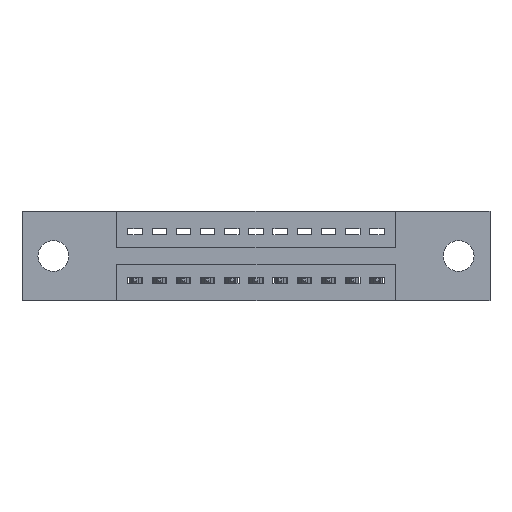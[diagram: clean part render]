
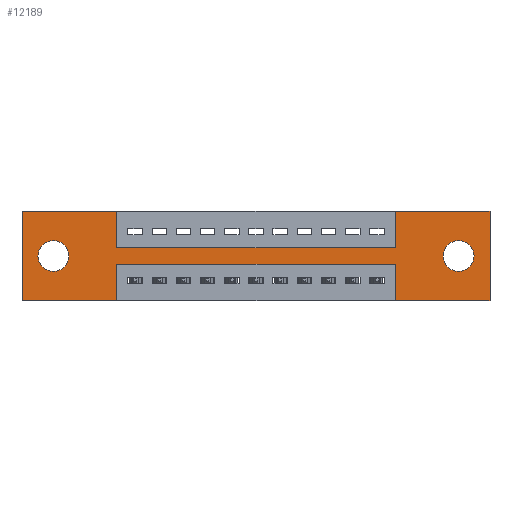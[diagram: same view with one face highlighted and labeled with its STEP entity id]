
A CAD part, front view. The second image highlights one B-rep face of the part: STEP entity #12189.
In plain terms, the highlighted planar face has unit normal (0, -1, 0).
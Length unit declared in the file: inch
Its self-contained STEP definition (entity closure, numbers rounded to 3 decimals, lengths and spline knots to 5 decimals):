
#134 = VERTEX_POINT ( 'NONE', #2562 ) ;
#169 = CARTESIAN_POINT ( 'NONE',  ( 0.3925, 0., -0.22 ) ) ;
#222 = DIRECTION ( 'NONE',  ( 0., 0., -1. ) ) ;
#341 = EDGE_CURVE ( 'NONE', #4711, #7004, #10070, .T. ) ;
#349 = ORIENTED_EDGE ( 'NONE', *, *, #8525, .F. ) ;
#428 = CARTESIAN_POINT ( 'NONE',  ( 1.935, 0., -0.37 ) ) ;
#443 = EDGE_LOOP ( 'NONE', ( #745, #349, #12490, #7075, #9271, #6505, #10443, #10310, #5885, #6499, #12311, #8963 ) ) ;
#560 = EDGE_CURVE ( 'NONE', #821, #6272, #3899, .T. ) ;
#649 = DIRECTION ( 'NONE',  ( 0., 0., 1. ) ) ;
#668 = CARTESIAN_POINT ( 'NONE',  ( 1.5425, 0., -0.37 ) ) ;
#745 = ORIENTED_EDGE ( 'NONE', *, *, #5936, .F. ) ;
#783 = DIRECTION ( 'NONE',  ( 0., 0., 1. ) ) ;
#821 = VERTEX_POINT ( 'NONE', #4050 ) ;
#855 = EDGE_CURVE ( 'NONE', #2214, #8982, #4069, .T. ) ;
#941 = AXIS2_PLACEMENT_3D ( 'NONE', #1010, #11714, #4969 ) ;
#1010 = CARTESIAN_POINT ( 'NONE',  ( 0.13, 0., -0.185 ) ) ;
#1178 = EDGE_CURVE ( 'NONE', #4798, #1387, #4210, .T. ) ;
#1194 = LINE ( 'NONE', #11105, #7691 ) ;
#1252 = VECTOR ( 'NONE', #10037, 39.37008 ) ;
#1342 = VECTOR ( 'NONE', #5977, 39.37008 ) ;
#1387 = VERTEX_POINT ( 'NONE', #1488 ) ;
#1488 = CARTESIAN_POINT ( 'NONE',  ( 1.5425, 0., 0. ) ) ;
#1522 = DIRECTION ( 'NONE',  ( 1., 0., 0. ) ) ;
#1753 = CARTESIAN_POINT ( 'NONE',  ( 1.5425, 0., 0. ) ) ;
#1761 = DIRECTION ( 'NONE',  ( -1., 0., 0. ) ) ;
#1895 = CARTESIAN_POINT ( 'NONE',  ( 1.805, 0., -0.121 ) ) ;
#2015 = VECTOR ( 'NONE', #1522, 39.37008 ) ;
#2032 = CARTESIAN_POINT ( 'NONE',  ( 1.5425, 0., -0.37 ) ) ;
#2048 = AXIS2_PLACEMENT_3D ( 'NONE', #8367, #9391, #8328 ) ;
#2094 = DIRECTION ( 'NONE',  ( -1., 0., 0. ) ) ;
#2175 = VECTOR ( 'NONE', #8903, 39.37008 ) ;
#2214 = VERTEX_POINT ( 'NONE', #9057 ) ;
#2562 = CARTESIAN_POINT ( 'NONE',  ( 1.935, 0., 0. ) ) ;
#2919 = CIRCLE ( 'NONE', #2048, 0.064 ) ;
#3237 = DIRECTION ( 'NONE',  ( 0., 0., -1. ) ) ;
#3252 = AXIS2_PLACEMENT_3D ( 'NONE', #12270, #11256, #649 ) ;
#3344 = VERTEX_POINT ( 'NONE', #7379 ) ;
#3412 = EDGE_CURVE ( 'NONE', #1387, #134, #9709, .T. ) ;
#3448 = FACE_OUTER_BOUND ( 'NONE', #443, .T. ) ;
#3622 = VERTEX_POINT ( 'NONE', #5799 ) ;
#3899 = LINE ( 'NONE', #12451, #10697 ) ;
#3951 = CARTESIAN_POINT ( 'NONE',  ( 1.935, 0., 0. ) ) ;
#4050 = CARTESIAN_POINT ( 'NONE',  ( 0., 0., 0. ) ) ;
#4065 = FACE_BOUND ( 'NONE', #8158, .T. ) ;
#4069 = CIRCLE ( 'NONE', #9921, 0.064 ) ;
#4089 = CARTESIAN_POINT ( 'NONE',  ( 0., 0., -0.37 ) ) ;
#4210 = LINE ( 'NONE', #1753, #8873 ) ;
#4297 = DIRECTION ( 'NONE',  ( 0., -1., 0. ) ) ;
#4382 = CIRCLE ( 'NONE', #941, 0.064 ) ;
#4503 = VECTOR ( 'NONE', #11838, 39.37008 ) ;
#4504 = DIRECTION ( 'NONE',  ( 0., 0., -1. ) ) ;
#4623 = CIRCLE ( 'NONE', #3252, 0.064 ) ;
#4711 = VERTEX_POINT ( 'NONE', #428 ) ;
#4733 = ORIENTED_EDGE ( 'NONE', *, *, #11001, .T. ) ;
#4798 = VERTEX_POINT ( 'NONE', #7018 ) ;
#4969 = DIRECTION ( 'NONE',  ( 0., 0., 1. ) ) ;
#5006 = EDGE_CURVE ( 'NONE', #5894, #9807, #5270, .T. ) ;
#5066 = CARTESIAN_POINT ( 'NONE',  ( 0.3925, 0., -0.37 ) ) ;
#5270 = LINE ( 'NONE', #12203, #12208 ) ;
#5799 = CARTESIAN_POINT ( 'NONE',  ( 0.3925, 0., -0.15 ) ) ;
#5836 = EDGE_CURVE ( 'NONE', #6272, #3622, #1194, .T. ) ;
#5843 = VECTOR ( 'NONE', #8838, 39.37008 ) ;
#5885 = ORIENTED_EDGE ( 'NONE', *, *, #5836, .F. ) ;
#5894 = VERTEX_POINT ( 'NONE', #5066 ) ;
#5936 = EDGE_CURVE ( 'NONE', #8462, #5894, #8294, .T. ) ;
#5956 = EDGE_LOOP ( 'NONE', ( #9849, #4733 ) ) ;
#5977 = DIRECTION ( 'NONE',  ( 0., 0., -1. ) ) ;
#6069 = CARTESIAN_POINT ( 'NONE',  ( 0.3925, 0., -0.37 ) ) ;
#6190 = CARTESIAN_POINT ( 'NONE',  ( 0.3925, 0., 0. ) ) ;
#6270 = LINE ( 'NONE', #169, #10777 ) ;
#6272 = VERTEX_POINT ( 'NONE', #6190 ) ;
#6487 = CARTESIAN_POINT ( 'NONE',  ( 0., 0., 0. ) ) ;
#6499 = ORIENTED_EDGE ( 'NONE', *, *, #560, .F. ) ;
#6505 = ORIENTED_EDGE ( 'NONE', *, *, #3412, .F. ) ;
#6520 = EDGE_CURVE ( 'NONE', #134, #4711, #10956, .T. ) ;
#6624 = VERTEX_POINT ( 'NONE', #7841 ) ;
#7004 = VERTEX_POINT ( 'NONE', #668 ) ;
#7018 = CARTESIAN_POINT ( 'NONE',  ( 1.5425, 0., -0.15 ) ) ;
#7023 = CARTESIAN_POINT ( 'NONE',  ( 0., 0., -0.37 ) ) ;
#7075 = ORIENTED_EDGE ( 'NONE', *, *, #341, .F. ) ;
#7157 = EDGE_CURVE ( 'NONE', #9807, #821, #8112, .T. ) ;
#7293 = CARTESIAN_POINT ( 'NONE',  ( 0., 0., 0. ) ) ;
#7379 = CARTESIAN_POINT ( 'NONE',  ( 0.13, 0., -0.249 ) ) ;
#7628 = LINE ( 'NONE', #2032, #2175 ) ;
#7691 = VECTOR ( 'NONE', #4504, 39.37008 ) ;
#7710 = CARTESIAN_POINT ( 'NONE',  ( 0.3925, 0., -0.22 ) ) ;
#7737 = CARTESIAN_POINT ( 'NONE',  ( 0., 0., -0.37 ) ) ;
#7841 = CARTESIAN_POINT ( 'NONE',  ( 1.5425, 0., -0.22 ) ) ;
#8112 = LINE ( 'NONE', #6487, #10029 ) ;
#8154 = FACE_BOUND ( 'NONE', #5956, .T. ) ;
#8158 = EDGE_LOOP ( 'NONE', ( #8286, #10782 ) ) ;
#8221 = EDGE_CURVE ( 'NONE', #7004, #6624, #7628, .T. ) ;
#8286 = ORIENTED_EDGE ( 'NONE', *, *, #9202, .T. ) ;
#8294 = LINE ( 'NONE', #6069, #1342 ) ;
#8328 = DIRECTION ( 'NONE',  ( 0., 0., -1. ) ) ;
#8349 = LINE ( 'NONE', #11939, #1252 ) ;
#8367 = CARTESIAN_POINT ( 'NONE',  ( 1.805, 0., -0.185 ) ) ;
#8375 = EDGE_CURVE ( 'NONE', #9333, #3344, #4623, .T. ) ;
#8462 = VERTEX_POINT ( 'NONE', #7710 ) ;
#8525 = EDGE_CURVE ( 'NONE', #6624, #8462, #6270, .T. ) ;
#8773 = AXIS2_PLACEMENT_3D ( 'NONE', #7023, #4297, #222 ) ;
#8838 = DIRECTION ( 'NONE',  ( 0., 0., -1. ) ) ;
#8873 = VECTOR ( 'NONE', #11440, 39.37008 ) ;
#8903 = DIRECTION ( 'NONE',  ( 0., 0., 1. ) ) ;
#8963 = ORIENTED_EDGE ( 'NONE', *, *, #5006, .F. ) ;
#8980 = DIRECTION ( 'NONE',  ( 0., 1., 0. ) ) ;
#8982 = VERTEX_POINT ( 'NONE', #1895 ) ;
#9057 = CARTESIAN_POINT ( 'NONE',  ( 1.805, 0., -0.249 ) ) ;
#9202 = EDGE_CURVE ( 'NONE', #8982, #2214, #2919, .T. ) ;
#9271 = ORIENTED_EDGE ( 'NONE', *, *, #6520, .F. ) ;
#9333 = VERTEX_POINT ( 'NONE', #11297 ) ;
#9391 = DIRECTION ( 'NONE',  ( 0., 1., 0. ) ) ;
#9709 = LINE ( 'NONE', #7293, #2015 ) ;
#9807 = VERTEX_POINT ( 'NONE', #7737 ) ;
#9849 = ORIENTED_EDGE ( 'NONE', *, *, #8375, .T. ) ;
#9921 = AXIS2_PLACEMENT_3D ( 'NONE', #11596, #8980, #3237 ) ;
#10026 = EDGE_CURVE ( 'NONE', #3622, #4798, #8349, .T. ) ;
#10029 = VECTOR ( 'NONE', #783, 39.37008 ) ;
#10037 = DIRECTION ( 'NONE',  ( 1., 0., 0. ) ) ;
#10070 = LINE ( 'NONE', #4089, #4503 ) ;
#10310 = ORIENTED_EDGE ( 'NONE', *, *, #10026, .F. ) ;
#10443 = ORIENTED_EDGE ( 'NONE', *, *, #1178, .F. ) ;
#10697 = VECTOR ( 'NONE', #12284, 39.37008 ) ;
#10777 = VECTOR ( 'NONE', #2094, 39.37008 ) ;
#10782 = ORIENTED_EDGE ( 'NONE', *, *, #855, .T. ) ;
#10956 = LINE ( 'NONE', #3951, #5843 ) ;
#11001 = EDGE_CURVE ( 'NONE', #3344, #9333, #4382, .T. ) ;
#11105 = CARTESIAN_POINT ( 'NONE',  ( 0.3925, 0., 0. ) ) ;
#11256 = DIRECTION ( 'NONE',  ( 0., 1., 0. ) ) ;
#11297 = CARTESIAN_POINT ( 'NONE',  ( 0.13, 0., -0.121 ) ) ;
#11440 = DIRECTION ( 'NONE',  ( 0., 0., 1. ) ) ;
#11596 = CARTESIAN_POINT ( 'NONE',  ( 1.805, 0., -0.185 ) ) ;
#11685 = PLANE ( 'NONE',  #8773 ) ;
#11714 = DIRECTION ( 'NONE',  ( 0., 1., 0. ) ) ;
#11838 = DIRECTION ( 'NONE',  ( -1., 0., 0. ) ) ;
#11939 = CARTESIAN_POINT ( 'NONE',  ( 0.3925, 0., -0.15 ) ) ;
#12189 = ADVANCED_FACE ( 'NONE', ( #4065, #8154, #3448 ), #11685, .T. ) ;
#12203 = CARTESIAN_POINT ( 'NONE',  ( 0., 0., -0.37 ) ) ;
#12208 = VECTOR ( 'NONE', #1761, 39.37008 ) ;
#12270 = CARTESIAN_POINT ( 'NONE',  ( 0.13, 0., -0.185 ) ) ;
#12284 = DIRECTION ( 'NONE',  ( 1., 0., 0. ) ) ;
#12311 = ORIENTED_EDGE ( 'NONE', *, *, #7157, .F. ) ;
#12451 = CARTESIAN_POINT ( 'NONE',  ( 0., 0., 0. ) ) ;
#12490 = ORIENTED_EDGE ( 'NONE', *, *, #8221, .F. ) ;
